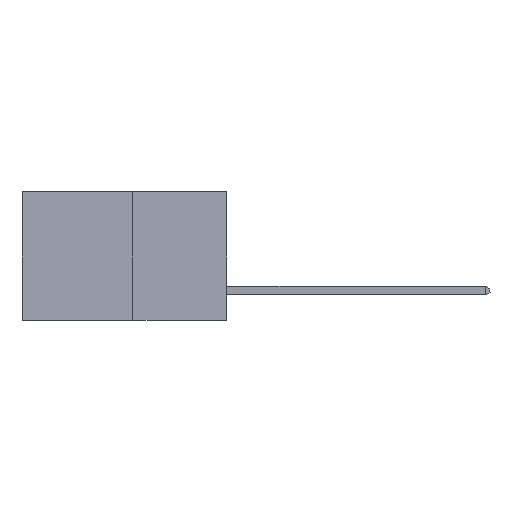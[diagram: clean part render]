
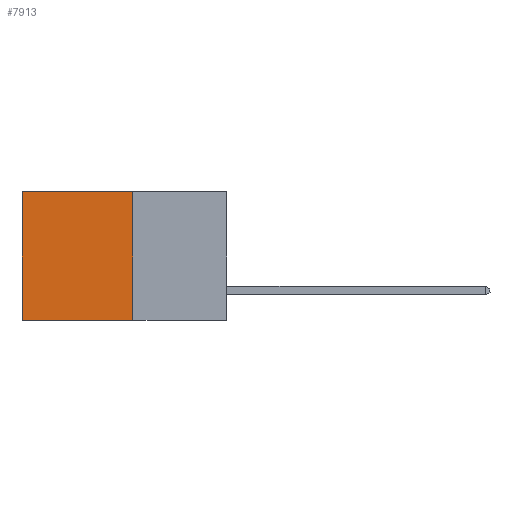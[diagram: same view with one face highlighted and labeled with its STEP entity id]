
A CAD part, left-side view. The second image highlights one B-rep face of the part: STEP entity #7913.
In plain terms, the highlighted planar face has unit normal (-1, 0, 0).
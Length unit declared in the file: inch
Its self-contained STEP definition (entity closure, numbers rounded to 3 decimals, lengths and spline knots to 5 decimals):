
#1362 = LINE ( 'NONE', #18421, #17200 ) ;
#1455 = CARTESIAN_POINT ( 'NONE',  ( 0.277, 0.27, -0.37 ) ) ;
#2773 = FACE_OUTER_BOUND ( 'NONE', #16221, .T. ) ;
#3025 = VERTEX_POINT ( 'NONE', #4996 ) ;
#3451 = CARTESIAN_POINT ( 'NONE',  ( 0.277, 0.59, -0.37 ) ) ;
#3764 = CARTESIAN_POINT ( 'NONE',  ( 0.277, 0.27, 0. ) ) ;
#4932 = AXIS2_PLACEMENT_3D ( 'NONE', #16033, #7153, #17460 ) ;
#4996 = CARTESIAN_POINT ( 'NONE',  ( 0.277, 0.59, 0. ) ) ;
#5392 = CARTESIAN_POINT ( 'NONE',  ( 0.277, 0.27, -0.37 ) ) ;
#6292 = LINE ( 'NONE', #8329, #17147 ) ;
#6463 = EDGE_CURVE ( 'NONE', #3025, #19194, #1362, .T. ) ;
#6834 = DIRECTION ( 'NONE',  ( 0., 1., 0. ) ) ;
#7153 = DIRECTION ( 'NONE',  ( 1., 0., 0. ) ) ;
#7580 = VERTEX_POINT ( 'NONE', #7880 ) ;
#7880 = CARTESIAN_POINT ( 'NONE',  ( 0.277, 0.27, 0. ) ) ;
#7913 = ADVANCED_FACE ( 'NONE', ( #2773 ), #13039, .F. ) ;
#8107 = DIRECTION ( 'NONE',  ( 0., 0., -1. ) ) ;
#8329 = CARTESIAN_POINT ( 'NONE',  ( 0.277, 0.27, -0.37 ) ) ;
#9011 = ORIENTED_EDGE ( 'NONE', *, *, #12378, .F. ) ;
#9402 = VECTOR ( 'NONE', #16348, 39.37008 ) ;
#10087 = EDGE_CURVE ( 'NONE', #7580, #3025, #10143, .T. ) ;
#10143 = LINE ( 'NONE', #3764, #18019 ) ;
#10596 = ORIENTED_EDGE ( 'NONE', *, *, #15499, .F. ) ;
#12201 = ORIENTED_EDGE ( 'NONE', *, *, #10087, .T. ) ;
#12378 = EDGE_CURVE ( 'NONE', #7580, #18102, #6292, .T. ) ;
#13039 = PLANE ( 'NONE',  #4932 ) ;
#13253 = ORIENTED_EDGE ( 'NONE', *, *, #6463, .T. ) ;
#15499 = EDGE_CURVE ( 'NONE', #18102, #19194, #17250, .T. ) ;
#15683 = DIRECTION ( 'NONE',  ( 0., 0., -1. ) ) ;
#16033 = CARTESIAN_POINT ( 'NONE',  ( 0.277, 0.27, -0.37 ) ) ;
#16221 = EDGE_LOOP ( 'NONE', ( #13253, #10596, #9011, #12201 ) ) ;
#16348 = DIRECTION ( 'NONE',  ( 0., 1., 0. ) ) ;
#17147 = VECTOR ( 'NONE', #15683, 39.37008 ) ;
#17200 = VECTOR ( 'NONE', #8107, 39.37008 ) ;
#17250 = LINE ( 'NONE', #1455, #9402 ) ;
#17460 = DIRECTION ( 'NONE',  ( 0., 0., -1. ) ) ;
#18019 = VECTOR ( 'NONE', #6834, 39.37008 ) ;
#18102 = VERTEX_POINT ( 'NONE', #5392 ) ;
#18421 = CARTESIAN_POINT ( 'NONE',  ( 0.277, 0.59, -0.37 ) ) ;
#19194 = VERTEX_POINT ( 'NONE', #3451 ) ;
